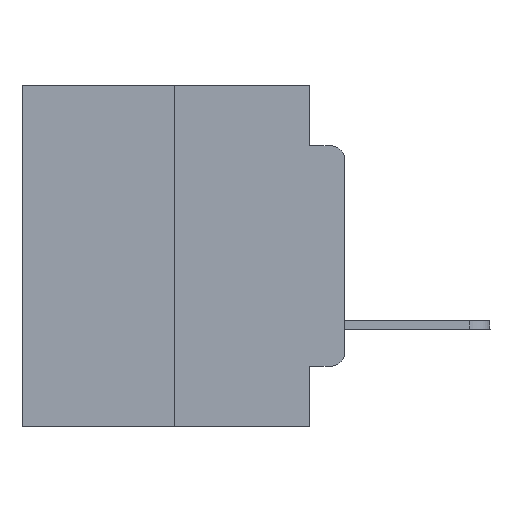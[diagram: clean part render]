
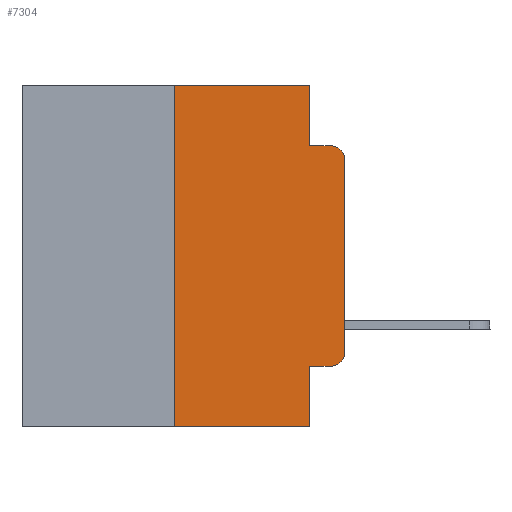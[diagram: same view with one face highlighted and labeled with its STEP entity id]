
A CAD part, left-side view. The second image highlights one B-rep face of the part: STEP entity #7304.
In plain terms, the highlighted planar face has unit normal (-1, 0, 0).
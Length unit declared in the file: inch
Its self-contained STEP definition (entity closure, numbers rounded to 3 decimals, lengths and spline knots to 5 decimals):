
#168 = CARTESIAN_POINT ( 'NONE',  ( 0., 0.02, -0.4115 ) ) ;
#593 = ORIENTED_EDGE ( 'NONE', *, *, #24217, .F. ) ;
#900 = ORIENTED_EDGE ( 'NONE', *, *, #4177, .T. ) ;
#1012 = VECTOR ( 'NONE', #9526, 39.37008 ) ;
#1048 = VERTEX_POINT ( 'NONE', #11086 ) ;
#1210 = DIRECTION ( 'NONE',  ( 0., 0., -1. ) ) ;
#1321 = ORIENTED_EDGE ( 'NONE', *, *, #10067, .F. ) ;
#1408 = EDGE_CURVE ( 'NONE', #4335, #7359, #11790, .T. ) ;
#2439 = CARTESIAN_POINT ( 'NONE',  ( 0., 0.02, -0.1085 ) ) ;
#2573 = LINE ( 'NONE', #25090, #21512 ) ;
#2771 = CARTESIAN_POINT ( 'NONE',  ( 0., 0.051, 0. ) ) ;
#3728 = PLANE ( 'NONE',  #7261 ) ;
#3760 = CARTESIAN_POINT ( 'NONE',  ( 0., 0., 0. ) ) ;
#3929 = DIRECTION ( 'NONE',  ( 0., -1., 0. ) ) ;
#4177 = EDGE_CURVE ( 'NONE', #1048, #12623, #6456, .T. ) ;
#4332 = ORIENTED_EDGE ( 'NONE', *, *, #12682, .T. ) ;
#4335 = VERTEX_POINT ( 'NONE', #17708 ) ;
#4460 = ORIENTED_EDGE ( 'NONE', *, *, #11264, .F. ) ;
#4513 = VERTEX_POINT ( 'NONE', #9807 ) ;
#6139 = VERTEX_POINT ( 'NONE', #13570 ) ;
#6452 = VECTOR ( 'NONE', #22672, 39.37008 ) ;
#6456 = LINE ( 'NONE', #16693, #6452 ) ;
#7261 = AXIS2_PLACEMENT_3D ( 'NONE', #22134, #13838, #18193 ) ;
#7304 = ADVANCED_FACE ( 'NONE', ( #9886 ), #3728, .F. ) ;
#7359 = VERTEX_POINT ( 'NONE', #7982 ) ;
#7598 = ORIENTED_EDGE ( 'NONE', *, *, #1408, .T. ) ;
#7982 = CARTESIAN_POINT ( 'NONE',  ( 0., 0.02, -0.0885 ) ) ;
#8098 = CIRCLE ( 'NONE', #15048, 0.02 ) ;
#9188 = VECTOR ( 'NONE', #24549, 39.37008 ) ;
#9277 = CARTESIAN_POINT ( 'NONE',  ( 0., 0.02, -0.3915 ) ) ;
#9477 = CARTESIAN_POINT ( 'NONE',  ( 0., 0.473, 0. ) ) ;
#9526 = DIRECTION ( 'NONE',  ( 0., 0., -1. ) ) ;
#9703 = CARTESIAN_POINT ( 'NONE',  ( 0., 0.051, -0.4115 ) ) ;
#9807 = CARTESIAN_POINT ( 'NONE',  ( 0., 0., -0.3915 ) ) ;
#9886 = FACE_OUTER_BOUND ( 'NONE', #23958, .T. ) ;
#10067 = EDGE_CURVE ( 'NONE', #18527, #13151, #23562, .T. ) ;
#10724 = VERTEX_POINT ( 'NONE', #168 ) ;
#10802 = DIRECTION ( 'NONE',  ( -1., 0., 0. ) ) ;
#10936 = DIRECTION ( 'NONE',  ( 0., 0., 1. ) ) ;
#11086 = CARTESIAN_POINT ( 'NONE',  ( 0., 0.25, -0.5 ) ) ;
#11264 = EDGE_CURVE ( 'NONE', #1048, #6139, #2573, .T. ) ;
#11790 = CIRCLE ( 'NONE', #18298, 0.02 ) ;
#12199 = ORIENTED_EDGE ( 'NONE', *, *, #17855, .T. ) ;
#12623 = VERTEX_POINT ( 'NONE', #22063 ) ;
#12682 = EDGE_CURVE ( 'NONE', #10724, #4513, #8098, .T. ) ;
#13151 = VERTEX_POINT ( 'NONE', #13873 ) ;
#13434 = DIRECTION ( 'NONE',  ( 0., 0., -1. ) ) ;
#13570 = CARTESIAN_POINT ( 'NONE',  ( 0., 0.25, 0. ) ) ;
#13838 = DIRECTION ( 'NONE',  ( 1., 0., 0. ) ) ;
#13873 = CARTESIAN_POINT ( 'NONE',  ( 0., 0.051, -0.0885 ) ) ;
#14209 = DIRECTION ( 'NONE',  ( 0., -1., 0. ) ) ;
#14684 = LINE ( 'NONE', #3760, #19144 ) ;
#15048 = AXIS2_PLACEMENT_3D ( 'NONE', #9277, #24244, #1210 ) ;
#16270 = LINE ( 'NONE', #16540, #9188 ) ;
#16540 = CARTESIAN_POINT ( 'NONE',  ( 0., 0.051, -0.0885 ) ) ;
#16693 = CARTESIAN_POINT ( 'NONE',  ( 0., 0.473, -0.5 ) ) ;
#16791 = VECTOR ( 'NONE', #13434, 39.37008 ) ;
#16884 = ORIENTED_EDGE ( 'NONE', *, *, #19677, .T. ) ;
#17402 = VECTOR ( 'NONE', #3929, 39.37008 ) ;
#17441 = CARTESIAN_POINT ( 'NONE',  ( 0., 0.051, 0. ) ) ;
#17708 = CARTESIAN_POINT ( 'NONE',  ( 0., 0., -0.1085 ) ) ;
#17855 = EDGE_CURVE ( 'NONE', #21696, #10724, #25055, .T. ) ;
#18193 = DIRECTION ( 'NONE',  ( 0., 0., -1. ) ) ;
#18298 = AXIS2_PLACEMENT_3D ( 'NONE', #2439, #10802, #20992 ) ;
#18527 = VERTEX_POINT ( 'NONE', #19026 ) ;
#18637 = DIRECTION ( 'NONE',  ( 0., 0., 1. ) ) ;
#18661 = CARTESIAN_POINT ( 'NONE',  ( 0., 0.051, -0.4115 ) ) ;
#19026 = CARTESIAN_POINT ( 'NONE',  ( 0., 0.051, 0. ) ) ;
#19052 = ORIENTED_EDGE ( 'NONE', *, *, #24054, .F. ) ;
#19144 = VECTOR ( 'NONE', #18637, 39.37008 ) ;
#19677 = EDGE_CURVE ( 'NONE', #4513, #4335, #14684, .T. ) ;
#20521 = EDGE_CURVE ( 'NONE', #13151, #7359, #16270, .T. ) ;
#20992 = DIRECTION ( 'NONE',  ( 0., 0., -1. ) ) ;
#21330 = LINE ( 'NONE', #2771, #16791 ) ;
#21512 = VECTOR ( 'NONE', #10936, 39.37008 ) ;
#21696 = VERTEX_POINT ( 'NONE', #9703 ) ;
#22063 = CARTESIAN_POINT ( 'NONE',  ( 0., 0.051, -0.5 ) ) ;
#22134 = CARTESIAN_POINT ( 'NONE',  ( 0., 0.473, 0. ) ) ;
#22672 = DIRECTION ( 'NONE',  ( 0., -1., 0. ) ) ;
#23349 = ORIENTED_EDGE ( 'NONE', *, *, #20521, .F. ) ;
#23562 = LINE ( 'NONE', #17441, #1012 ) ;
#23958 = EDGE_LOOP ( 'NONE', ( #16884, #7598, #23349, #1321, #593, #4460, #900, #19052, #12199, #4332 ) ) ;
#24054 = EDGE_CURVE ( 'NONE', #21696, #12623, #21330, .T. ) ;
#24217 = EDGE_CURVE ( 'NONE', #6139, #18527, #24546, .T. ) ;
#24244 = DIRECTION ( 'NONE',  ( -1., 0., 0. ) ) ;
#24546 = LINE ( 'NONE', #9477, #24587 ) ;
#24549 = DIRECTION ( 'NONE',  ( 0., -1., 0. ) ) ;
#24587 = VECTOR ( 'NONE', #14209, 39.37008 ) ;
#25055 = LINE ( 'NONE', #18661, #17402 ) ;
#25090 = CARTESIAN_POINT ( 'NONE',  ( 0., 0.25, 0. ) ) ;
